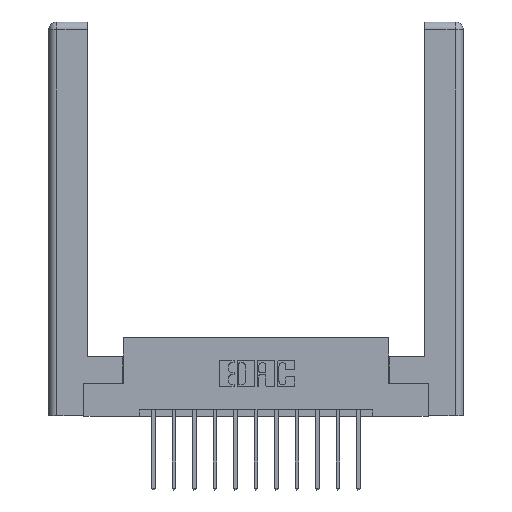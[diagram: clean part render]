
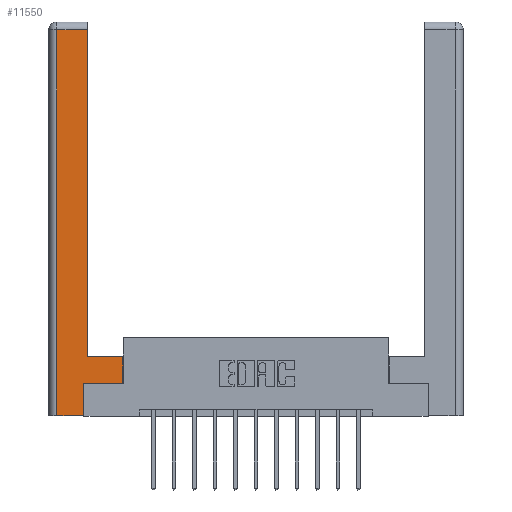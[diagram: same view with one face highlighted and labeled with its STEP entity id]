
A CAD part, top view. The second image highlights one B-rep face of the part: STEP entity #11550.
In plain terms, the highlighted planar face has unit normal (0, 0, 1).
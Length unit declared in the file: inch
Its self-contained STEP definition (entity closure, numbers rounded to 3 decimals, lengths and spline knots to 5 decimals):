
#176 = VERTEX_POINT ( 'NONE', #13461 ) ;
#296 = EDGE_CURVE ( 'NONE', #4486, #14346, #10831, .T. ) ;
#482 = CARTESIAN_POINT ( 'NONE',  ( 0.295, 2.94, 0. ) ) ;
#805 = DIRECTION ( 'NONE',  ( -1., 0., 0. ) ) ;
#1036 = ORIENTED_EDGE ( 'NONE', *, *, #12647, .T. ) ;
#1086 = DIRECTION ( 'NONE',  ( 0., 0., -1. ) ) ;
#1132 = ORIENTED_EDGE ( 'NONE', *, *, #1183, .T. ) ;
#1183 = EDGE_CURVE ( 'NONE', #14346, #10591, #8531, .T. ) ;
#1556 = DIRECTION ( 'NONE',  ( -1., 0., 0. ) ) ;
#1683 = ORIENTED_EDGE ( 'NONE', *, *, #11988, .T. ) ;
#1924 = LINE ( 'NONE', #14876, #7757 ) ;
#1960 = DIRECTION ( 'NONE',  ( 0., -1., 0. ) ) ;
#2217 = VECTOR ( 'NONE', #12488, 39.37008 ) ;
#2383 = CARTESIAN_POINT ( 'NONE',  ( 0., 0., 0. ) ) ;
#2389 = ORIENTED_EDGE ( 'NONE', *, *, #14371, .T. ) ;
#3086 = ORIENTED_EDGE ( 'NONE', *, *, #12686, .T. ) ;
#3200 = CARTESIAN_POINT ( 'NONE',  ( 0.265, 0.245, 0. ) ) ;
#3243 = CARTESIAN_POINT ( 'NONE',  ( 0.265, 0.245, 0. ) ) ;
#3253 = VERTEX_POINT ( 'NONE', #8606 ) ;
#3818 = CARTESIAN_POINT ( 'NONE',  ( 0.295, 0.45, 0. ) ) ;
#4046 = VERTEX_POINT ( 'NONE', #3200 ) ;
#4403 = CARTESIAN_POINT ( 'NONE',  ( 0.565, 0.245, 0. ) ) ;
#4486 = VERTEX_POINT ( 'NONE', #4766 ) ;
#4766 = CARTESIAN_POINT ( 'NONE',  ( 0.565, 0.245, 0. ) ) ;
#4915 = CARTESIAN_POINT ( 'NONE',  ( 0.0615, 2.94, 0. ) ) ;
#4983 = AXIS2_PLACEMENT_3D ( 'NONE', #2383, #1086, #10615 ) ;
#5193 = LINE ( 'NONE', #4915, #12587 ) ;
#5198 = VECTOR ( 'NONE', #1960, 39.37008 ) ;
#5607 = DIRECTION ( 'NONE',  ( 1., 0., 0. ) ) ;
#5801 = ORIENTED_EDGE ( 'NONE', *, *, #9013, .T. ) ;
#5862 = DIRECTION ( 'NONE',  ( 1., 0., 0. ) ) ;
#7345 = DIRECTION ( 'NONE',  ( 0., 1., 0. ) ) ;
#7584 = LINE ( 'NONE', #4403, #9618 ) ;
#7757 = VECTOR ( 'NONE', #5607, 39.37008 ) ;
#8531 = LINE ( 'NONE', #12618, #10369 ) ;
#8606 = CARTESIAN_POINT ( 'NONE',  ( 0.265, 0., 0. ) ) ;
#8711 = FACE_OUTER_BOUND ( 'NONE', #10311, .T. ) ;
#9013 = EDGE_CURVE ( 'NONE', #9751, #11984, #5193, .T. ) ;
#9325 = ORIENTED_EDGE ( 'NONE', *, *, #296, .T. ) ;
#9560 = EDGE_CURVE ( 'NONE', #4046, #4486, #7584, .T. ) ;
#9618 = VECTOR ( 'NONE', #5862, 39.37008 ) ;
#9751 = VERTEX_POINT ( 'NONE', #482 ) ;
#10311 = EDGE_LOOP ( 'NONE', ( #2389, #5801, #1683, #3086, #1036, #11678, #9325, #1132 ) ) ;
#10369 = VECTOR ( 'NONE', #805, 39.37008 ) ;
#10591 = VERTEX_POINT ( 'NONE', #3818 ) ;
#10615 = DIRECTION ( 'NONE',  ( -1., 0., 0. ) ) ;
#10798 = CARTESIAN_POINT ( 'NONE',  ( 0.565, 0.45, 0. ) ) ;
#10831 = LINE ( 'NONE', #11201, #2217 ) ;
#10880 = LINE ( 'NONE', #3243, #13311 ) ;
#11201 = CARTESIAN_POINT ( 'NONE',  ( 0.565, 0.45, 0. ) ) ;
#11282 = LINE ( 'NONE', #13731, #5198 ) ;
#11487 = DIRECTION ( 'NONE',  ( 0., 1., 0. ) ) ;
#11550 = ADVANCED_FACE ( 'NONE', ( #8711 ), #11723, .F. ) ;
#11678 = ORIENTED_EDGE ( 'NONE', *, *, #9560, .T. ) ;
#11723 = PLANE ( 'NONE',  #4983 ) ;
#11793 = LINE ( 'NONE', #12039, #15078 ) ;
#11984 = VERTEX_POINT ( 'NONE', #12522 ) ;
#11988 = EDGE_CURVE ( 'NONE', #11984, #176, #11282, .T. ) ;
#12039 = CARTESIAN_POINT ( 'NONE',  ( 0.295, 3., 0. ) ) ;
#12488 = DIRECTION ( 'NONE',  ( 0., 1., 0. ) ) ;
#12522 = CARTESIAN_POINT ( 'NONE',  ( 0.0615, 2.94, 0. ) ) ;
#12587 = VECTOR ( 'NONE', #1556, 39.37008 ) ;
#12618 = CARTESIAN_POINT ( 'NONE',  ( 0.295, 0.45, 0. ) ) ;
#12647 = EDGE_CURVE ( 'NONE', #3253, #4046, #10880, .T. ) ;
#12686 = EDGE_CURVE ( 'NONE', #176, #3253, #1924, .T. ) ;
#13311 = VECTOR ( 'NONE', #11487, 39.37008 ) ;
#13461 = CARTESIAN_POINT ( 'NONE',  ( 0.0615, 0., 0. ) ) ;
#13731 = CARTESIAN_POINT ( 'NONE',  ( 0.0615, 0., 0. ) ) ;
#14346 = VERTEX_POINT ( 'NONE', #10798 ) ;
#14371 = EDGE_CURVE ( 'NONE', #10591, #9751, #11793, .T. ) ;
#14876 = CARTESIAN_POINT ( 'NONE',  ( 0.265, 0., 0. ) ) ;
#15078 = VECTOR ( 'NONE', #7345, 39.37008 ) ;
